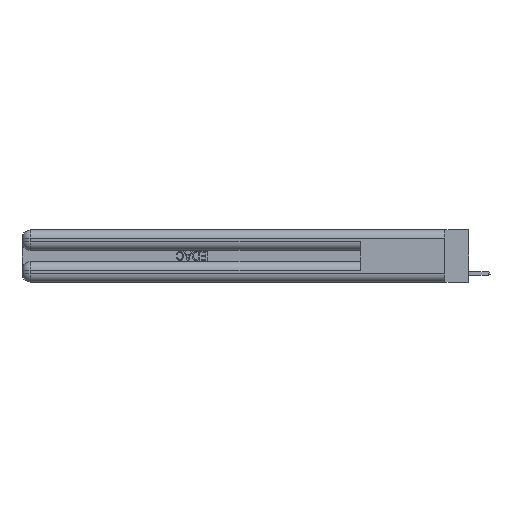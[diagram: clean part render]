
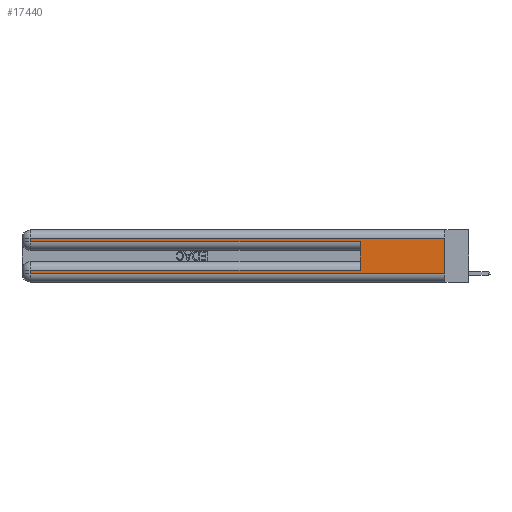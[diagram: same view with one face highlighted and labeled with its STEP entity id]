
A CAD part, left-side view. The second image highlights one B-rep face of the part: STEP entity #17440.
In plain terms, the highlighted planar face has unit normal (-1, 0, 0).
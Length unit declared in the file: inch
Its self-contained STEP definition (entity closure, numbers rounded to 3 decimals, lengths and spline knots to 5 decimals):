
#339 = CARTESIAN_POINT ( 'NONE',  ( 0., 0., 0.06 ) ) ;
#585 = DIRECTION ( 'NONE',  ( 0., 0., -1. ) ) ;
#1109 = CARTESIAN_POINT ( 'NONE',  ( 0., 2.94, 0.31 ) ) ;
#1113 = CARTESIAN_POINT ( 'NONE',  ( 0., 0.6, 0.285 ) ) ;
#1201 = LINE ( 'NONE', #9227, #6319 ) ;
#1708 = CARTESIAN_POINT ( 'NONE',  ( 0., 0.6, 0.145 ) ) ;
#1887 = CARTESIAN_POINT ( 'NONE',  ( 0., 0., 0.31 ) ) ;
#1942 = CARTESIAN_POINT ( 'NONE',  ( 0., 2.94, 0.06 ) ) ;
#2221 = ORIENTED_EDGE ( 'NONE', *, *, #25130, .T. ) ;
#4180 = ORIENTED_EDGE ( 'NONE', *, *, #24252, .T. ) ;
#4253 = EDGE_CURVE ( 'NONE', #5804, #14153, #12631, .T. ) ;
#4739 = LINE ( 'NONE', #6665, #20931 ) ;
#5606 = CARTESIAN_POINT ( 'NONE',  ( 0., 0., 0.085 ) ) ;
#5663 = EDGE_CURVE ( 'NONE', #26799, #5742, #4739, .T. ) ;
#5742 = VERTEX_POINT ( 'NONE', #18322 ) ;
#5804 = VERTEX_POINT ( 'NONE', #1942 ) ;
#5974 = PLANE ( 'NONE',  #16959 ) ;
#6143 = VERTEX_POINT ( 'NONE', #7173 ) ;
#6196 = VECTOR ( 'NONE', #23757, 39.37008 ) ;
#6319 = VECTOR ( 'NONE', #13669, 39.37008 ) ;
#6432 = ORIENTED_EDGE ( 'NONE', *, *, #5663, .T. ) ;
#6665 = CARTESIAN_POINT ( 'NONE',  ( 0., 2.94, 0.37 ) ) ;
#7173 = CARTESIAN_POINT ( 'NONE',  ( 0., 0.6, 0.085 ) ) ;
#8791 = EDGE_CURVE ( 'NONE', #6143, #16105, #9214, .T. ) ;
#9214 = LINE ( 'NONE', #1708, #20328 ) ;
#9227 = CARTESIAN_POINT ( 'NONE',  ( 0., 0., 0.285 ) ) ;
#9612 = LINE ( 'NONE', #5606, #10653 ) ;
#9831 = LINE ( 'NONE', #18307, #12483 ) ;
#9983 = CARTESIAN_POINT ( 'NONE',  ( 0., 0., 0.37 ) ) ;
#10257 = FACE_OUTER_BOUND ( 'NONE', #11231, .T. ) ;
#10653 = VECTOR ( 'NONE', #26561, 39.37008 ) ;
#11004 = ORIENTED_EDGE ( 'NONE', *, *, #12472, .F. ) ;
#11101 = ORIENTED_EDGE ( 'NONE', *, *, #4253, .T. ) ;
#11231 = EDGE_LOOP ( 'NONE', ( #11004, #19684, #6432, #4180, #27002, #12552, #2221, #11101 ) ) ;
#12472 = EDGE_CURVE ( 'NONE', #25534, #14153, #17502, .T. ) ;
#12483 = VECTOR ( 'NONE', #16629, 39.37008 ) ;
#12552 = ORIENTED_EDGE ( 'NONE', *, *, #22894, .T. ) ;
#12631 = LINE ( 'NONE', #14719, #15519 ) ;
#13584 = DIRECTION ( 'NONE',  ( 0., 0., -1. ) ) ;
#13656 = DIRECTION ( 'NONE',  ( 0., 0., 1. ) ) ;
#13669 = DIRECTION ( 'NONE',  ( 0., -1., 0. ) ) ;
#13729 = VECTOR ( 'NONE', #585, 39.37008 ) ;
#14153 = VERTEX_POINT ( 'NONE', #339 ) ;
#14453 = DIRECTION ( 'NONE',  ( 0., -1., 0. ) ) ;
#14719 = CARTESIAN_POINT ( 'NONE',  ( 0., 0., 0.06 ) ) ;
#15519 = VECTOR ( 'NONE', #14453, 39.37008 ) ;
#16042 = CARTESIAN_POINT ( 'NONE',  ( 0., 0., 0.31 ) ) ;
#16105 = VERTEX_POINT ( 'NONE', #1113 ) ;
#16580 = LINE ( 'NONE', #1887, #6196 ) ;
#16629 = DIRECTION ( 'NONE',  ( 0., 0., -1. ) ) ;
#16959 = AXIS2_PLACEMENT_3D ( 'NONE', #9983, #20952, #25252 ) ;
#17440 = ADVANCED_FACE ( 'NONE', ( #10257 ), #5974, .F. ) ;
#17502 = LINE ( 'NONE', #19598, #13729 ) ;
#18307 = CARTESIAN_POINT ( 'NONE',  ( 0., 2.94, 0.37 ) ) ;
#18322 = CARTESIAN_POINT ( 'NONE',  ( 0., 2.94, 0.285 ) ) ;
#19053 = VERTEX_POINT ( 'NONE', #21197 ) ;
#19598 = CARTESIAN_POINT ( 'NONE',  ( 0., 0., 0.37 ) ) ;
#19684 = ORIENTED_EDGE ( 'NONE', *, *, #21295, .T. ) ;
#20328 = VECTOR ( 'NONE', #13656, 39.37008 ) ;
#20931 = VECTOR ( 'NONE', #13584, 39.37008 ) ;
#20952 = DIRECTION ( 'NONE',  ( 1., 0., 0. ) ) ;
#21197 = CARTESIAN_POINT ( 'NONE',  ( 0., 2.94, 0.085 ) ) ;
#21295 = EDGE_CURVE ( 'NONE', #25534, #26799, #16580, .T. ) ;
#22894 = EDGE_CURVE ( 'NONE', #6143, #19053, #9612, .T. ) ;
#23757 = DIRECTION ( 'NONE',  ( 0., 1., 0. ) ) ;
#24252 = EDGE_CURVE ( 'NONE', #5742, #16105, #1201, .T. ) ;
#25130 = EDGE_CURVE ( 'NONE', #19053, #5804, #9831, .T. ) ;
#25252 = DIRECTION ( 'NONE',  ( 0., 0., -1. ) ) ;
#25534 = VERTEX_POINT ( 'NONE', #16042 ) ;
#26561 = DIRECTION ( 'NONE',  ( 0., 1., 0. ) ) ;
#26799 = VERTEX_POINT ( 'NONE', #1109 ) ;
#27002 = ORIENTED_EDGE ( 'NONE', *, *, #8791, .F. ) ;
